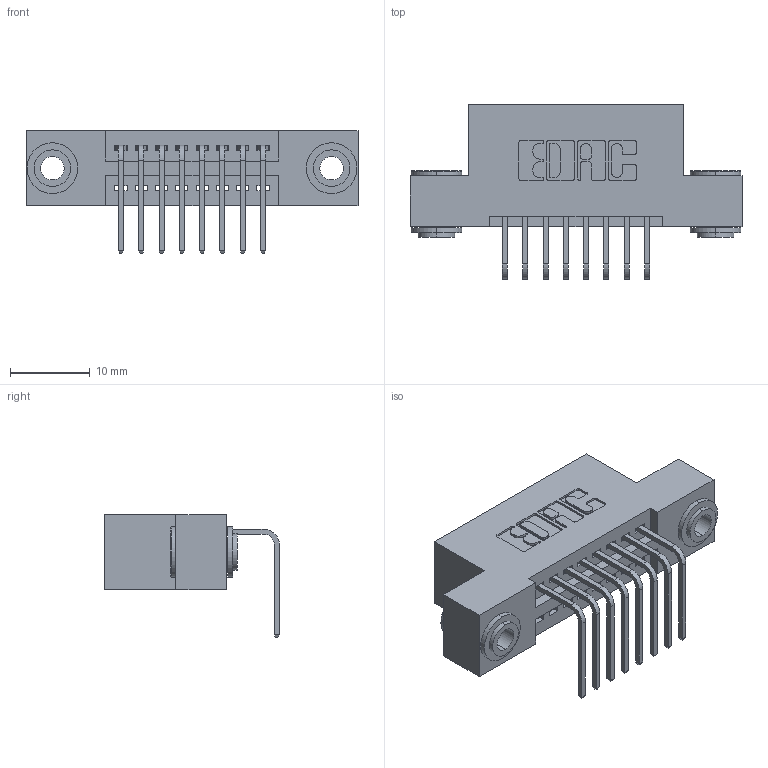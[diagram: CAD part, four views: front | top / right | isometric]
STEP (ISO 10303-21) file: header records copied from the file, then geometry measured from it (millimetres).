
FILE_DESCRIPTION (( 'STEP AP203' ), '1' );
FILE_NAME ('345-008-558-103.STEP', '2018-08-17T04:48:56', ( '' ), ( '' ), 'SwSTEP 2.0', 'SolidWorks 2016', '' );
FILE_SCHEMA (( 'CONFIG_CONTROL_DESIGN' ));
Length unit declared in the file: inch
Products named in the file (4): 345-292-001_558 Tail - 2; 345-250-002_345-250-002-102; 345-008-558-103; 345 Part_Flush Mounting Lugs - 0.156 Dia-TH
Assembly tree (11 placements, depth 2):
  345-008-558-103
    345 Part_Flush Mounting Lugs - 0.156 Dia-TH
    345-292-001_558 Tail - 2  x8
    345-250-002_345-250-002-102  x2
Bounding box: 41.53 x 21.83 x 15.37 mm (x, y, z)
Volume: 3712 mm3; surface area: 4841.9 mm2
Topology: 11 solids, 11 shells, 644 faces, 1873 edges, 1234 vertices
Faces by surface type: plane 426, cylinder 210, cone 8
Entity records: 11332 total; most frequent: CARTESIAN_POINT 1943, ORIENTED_EDGE 1878, DIRECTION 1777, EDGE_CURVE 939, LINE 751, VECTOR 751, VERTEX_POINT 622, AXIS2_PLACEMENT_3D 513
